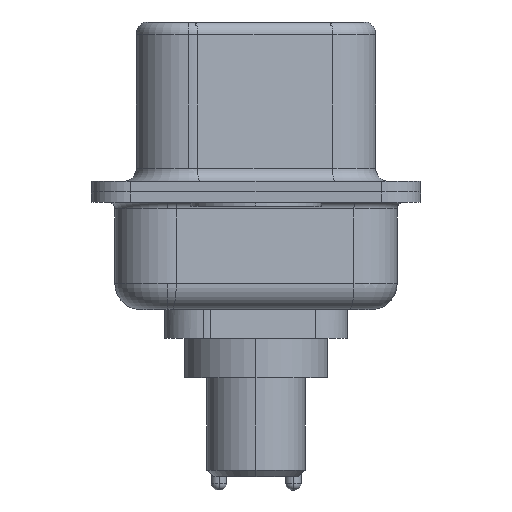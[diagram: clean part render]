
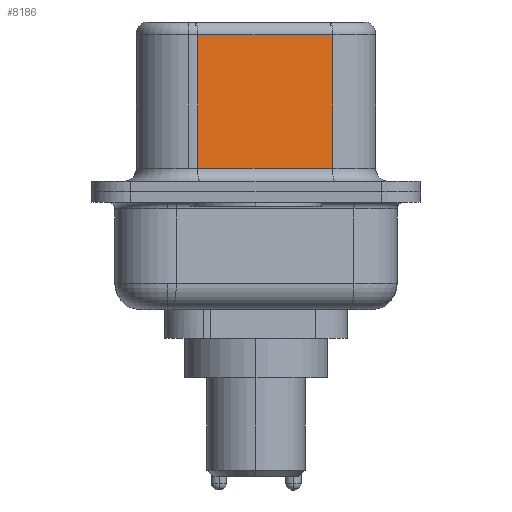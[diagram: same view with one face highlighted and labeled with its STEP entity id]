
A CAD part, left-side view. The second image highlights one B-rep face of the part: STEP entity #8186.
In plain terms, the highlighted planar face has unit normal (-0.985, -0.174, 0).
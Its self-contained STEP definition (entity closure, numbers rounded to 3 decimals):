
#252 = LINE ( 'NONE', #14734, #8527 ) ;
#2804 = VERTEX_POINT ( 'NONE', #11320 ) ;
#2882 = PLANE ( 'NONE',  #4761 ) ;
#3845 = CARTESIAN_POINT ( 'NONE',  ( 4.58, -2.927, 0.9 ) ) ;
#4388 = CARTESIAN_POINT ( 'NONE',  ( 4.58, -2.927, 6.02 ) ) ;
#4761 = AXIS2_PLACEMENT_3D ( 'NONE', #9388, #17629, #7846 ) ;
#5601 = VECTOR ( 'NONE', #11557, 1000. ) ;
#5968 = ORIENTED_EDGE ( 'NONE', *, *, #8347, .T. ) ;
#6773 = CARTESIAN_POINT ( 'NONE',  ( 4.58, -2.927, 6.52 ) ) ;
#7846 = DIRECTION ( 'NONE',  ( -0.174, 0.985, 0. ) ) ;
#8186 = ADVANCED_FACE ( 'NONE', ( #8982 ), #2882, .F. ) ;
#8347 = EDGE_CURVE ( 'NONE', #18070, #17746, #10463, .T. ) ;
#8527 = VECTOR ( 'NONE', #16426, 1000. ) ;
#8982 = FACE_OUTER_BOUND ( 'NONE', #14666, .T. ) ;
#9388 = CARTESIAN_POINT ( 'NONE',  ( 4.58, -2.927, 6.52 ) ) ;
#9683 = EDGE_CURVE ( 'NONE', #2804, #19875, #16351, .T. ) ;
#10463 = LINE ( 'NONE', #14706, #18773 ) ;
#11320 = CARTESIAN_POINT ( 'NONE',  ( 3.67, 2.233, 0.9 ) ) ;
#11557 = DIRECTION ( 'NONE',  ( 0., 0., -1. ) ) ;
#11921 = VECTOR ( 'NONE', #20251, 1000. ) ;
#13720 = CARTESIAN_POINT ( 'NONE',  ( 3.67, 2.233, 6.02 ) ) ;
#14182 = LINE ( 'NONE', #6773, #5601 ) ;
#14666 = EDGE_LOOP ( 'NONE', ( #15151, #5968, #20386, #19649 ) ) ;
#14706 = CARTESIAN_POINT ( 'NONE',  ( 4.58, -2.927, 6.02 ) ) ;
#14734 = CARTESIAN_POINT ( 'NONE',  ( 3.67, 2.233, 6.52 ) ) ;
#15151 = ORIENTED_EDGE ( 'NONE', *, *, #18942, .F. ) ;
#16351 = LINE ( 'NONE', #3845, #11921 ) ;
#16388 = DIRECTION ( 'NONE',  ( -0.174, 0.985, 0. ) ) ;
#16426 = DIRECTION ( 'NONE',  ( 0., 0., -1. ) ) ;
#17629 = DIRECTION ( 'NONE',  ( 0.985, 0.174, 0. ) ) ;
#17746 = VERTEX_POINT ( 'NONE', #13720 ) ;
#18070 = VERTEX_POINT ( 'NONE', #4388 ) ;
#18773 = VECTOR ( 'NONE', #16388, 1000. ) ;
#18942 = EDGE_CURVE ( 'NONE', #18070, #19875, #14182, .T. ) ;
#19175 = CARTESIAN_POINT ( 'NONE',  ( 4.58, -2.927, 0.9 ) ) ;
#19649 = ORIENTED_EDGE ( 'NONE', *, *, #9683, .T. ) ;
#19875 = VERTEX_POINT ( 'NONE', #19175 ) ;
#20251 = DIRECTION ( 'NONE',  ( 0.174, -0.985, 0. ) ) ;
#20386 = ORIENTED_EDGE ( 'NONE', *, *, #21134, .T. ) ;
#21134 = EDGE_CURVE ( 'NONE', #17746, #2804, #252, .T. ) ;
